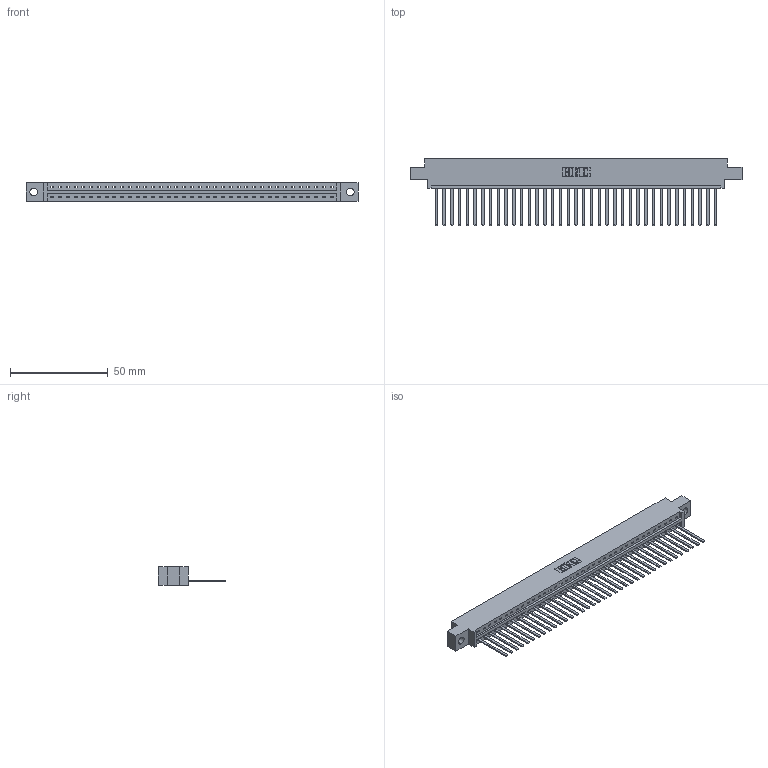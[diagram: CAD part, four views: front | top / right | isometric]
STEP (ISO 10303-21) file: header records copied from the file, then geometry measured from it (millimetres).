
FILE_DESCRIPTION (( 'STEP AP203' ), '1' );
FILE_NAME ('337-037-544-604.STEP', '2018-08-08T01:58:06', ( '' ), ( '' ), 'SwSTEP 2.0', 'SolidWorks 2016', '' );
FILE_SCHEMA (( 'CONFIG_CONTROL_DESIGN' ));
Length unit declared in the file: inch
Products named in the file (3): 337 Part_0.170 Offset - 0.156 Dia-TH; 345-292-001_345-293-144; 337-037-544-604
Assembly tree (38 placements, depth 2):
  337-037-544-604
    337 Part_0.170 Offset - 0.156 Dia-TH
    345-292-001_345-293-144  x37
Bounding box: 169.62 x 34.3 x 9.4 mm (x, y, z)
Volume: 17789.9 mm3; surface area: 19656.7 mm2
Topology: 38 solids, 38 shells, 2190 faces, 6613 edges, 4358 vertices
Faces by surface type: plane 1628, cylinder 562
Entity records: 28101 total; most frequent: CARTESIAN_POINT 4901, ORIENTED_EDGE 4874, DIRECTION 4131, EDGE_CURVE 2437, VECTOR 2313, LINE 2313, VERTEX_POINT 1622, AXIS2_PLACEMENT_3D 909
